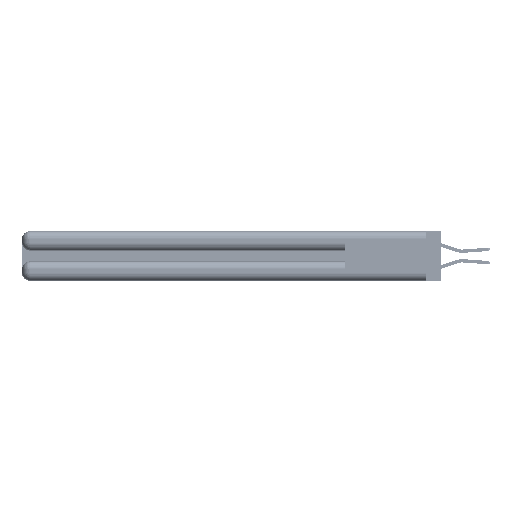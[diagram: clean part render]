
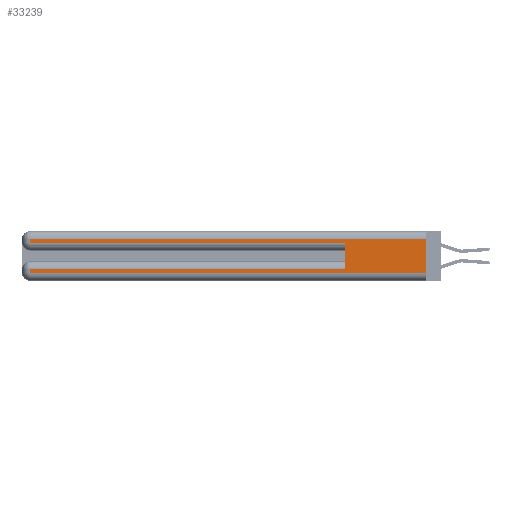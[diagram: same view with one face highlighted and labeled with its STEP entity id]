
A CAD part, left-side view. The second image highlights one B-rep face of the part: STEP entity #33239.
In plain terms, the highlighted planar face has unit normal (-1, 0, 0).
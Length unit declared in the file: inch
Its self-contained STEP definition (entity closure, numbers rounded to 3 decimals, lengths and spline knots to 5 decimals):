
#324 = LINE ( 'NONE', #23147, #6825 ) ;
#1380 = PLANE ( 'NONE',  #4083 ) ;
#4083 = AXIS2_PLACEMENT_3D ( 'NONE', #9706, #13821, #17948 ) ;
#4121 = CARTESIAN_POINT ( 'NONE',  ( 0., 0., 0.285 ) ) ;
#4352 = EDGE_CURVE ( 'NONE', #18697, #49655, #17958, .T. ) ;
#6003 = CARTESIAN_POINT ( 'NONE',  ( 0., 2.94, 0.085 ) ) ;
#6825 = VECTOR ( 'NONE', #51943, 39.37008 ) ;
#7717 = VERTEX_POINT ( 'NONE', #25868 ) ;
#7947 = LINE ( 'NONE', #16508, #23397 ) ;
#8087 = ORIENTED_EDGE ( 'NONE', *, *, #45344, .T. ) ;
#8477 = LINE ( 'NONE', #27884, #30405 ) ;
#9000 = VERTEX_POINT ( 'NONE', #42973 ) ;
#9706 = CARTESIAN_POINT ( 'NONE',  ( 0., 0., 0.37 ) ) ;
#9936 = VERTEX_POINT ( 'NONE', #25218 ) ;
#11226 = CARTESIAN_POINT ( 'NONE',  ( 0., 2.94, 0.285 ) ) ;
#11917 = DIRECTION ( 'NONE',  ( 0., 0., -1. ) ) ;
#12040 = ORIENTED_EDGE ( 'NONE', *, *, #44497, .T. ) ;
#12466 = EDGE_CURVE ( 'NONE', #9000, #18697, #31203, .T. ) ;
#12529 = EDGE_LOOP ( 'NONE', ( #28796, #12040, #33891, #22544, #28391, #52327, #8087, #31484 ) ) ;
#12564 = LINE ( 'NONE', #38827, #42848 ) ;
#13821 = DIRECTION ( 'NONE',  ( 1., 0., 0. ) ) ;
#16216 = CARTESIAN_POINT ( 'NONE',  ( 0., 2.94, 0.37 ) ) ;
#16252 = EDGE_CURVE ( 'NONE', #9936, #47673, #8477, .T. ) ;
#16508 = CARTESIAN_POINT ( 'NONE',  ( 0., 0.6, 0.145 ) ) ;
#17948 = DIRECTION ( 'NONE',  ( 0., 0., -1. ) ) ;
#17958 = LINE ( 'NONE', #4121, #23748 ) ;
#18697 = VERTEX_POINT ( 'NONE', #11226 ) ;
#19847 = LINE ( 'NONE', #52032, #21826 ) ;
#20217 = VECTOR ( 'NONE', #26576, 39.37008 ) ;
#21826 = VECTOR ( 'NONE', #31521, 39.37008 ) ;
#22544 = ORIENTED_EDGE ( 'NONE', *, *, #4352, .T. ) ;
#22994 = DIRECTION ( 'NONE',  ( 0., 1., 0. ) ) ;
#23147 = CARTESIAN_POINT ( 'NONE',  ( 0., 0., 0.085 ) ) ;
#23397 = VECTOR ( 'NONE', #37931, 39.37008 ) ;
#23748 = VECTOR ( 'NONE', #41397, 39.37008 ) ;
#25218 = CARTESIAN_POINT ( 'NONE',  ( 0., 0., 0.31 ) ) ;
#25563 = EDGE_CURVE ( 'NONE', #47698, #49655, #7947, .T. ) ;
#25868 = CARTESIAN_POINT ( 'NONE',  ( 0., 2.94, 0.06 ) ) ;
#26576 = DIRECTION ( 'NONE',  ( 0., 0., -1. ) ) ;
#27884 = CARTESIAN_POINT ( 'NONE',  ( 0., 0., 0.37 ) ) ;
#28391 = ORIENTED_EDGE ( 'NONE', *, *, #25563, .F. ) ;
#28796 = ORIENTED_EDGE ( 'NONE', *, *, #16252, .F. ) ;
#29294 = CARTESIAN_POINT ( 'NONE',  ( 0., 0.6, 0.085 ) ) ;
#30405 = VECTOR ( 'NONE', #48243, 39.37008 ) ;
#31203 = LINE ( 'NONE', #46912, #20217 ) ;
#31484 = ORIENTED_EDGE ( 'NONE', *, *, #49767, .T. ) ;
#31521 = DIRECTION ( 'NONE',  ( 0., -1., 0. ) ) ;
#32167 = EDGE_CURVE ( 'NONE', #47698, #36708, #324, .T. ) ;
#33239 = ADVANCED_FACE ( 'NONE', ( #45410 ), #1380, .F. ) ;
#33891 = ORIENTED_EDGE ( 'NONE', *, *, #12466, .T. ) ;
#36708 = VERTEX_POINT ( 'NONE', #6003 ) ;
#37908 = CARTESIAN_POINT ( 'NONE',  ( 0., 0., 0.06 ) ) ;
#37931 = DIRECTION ( 'NONE',  ( 0., 0., 1. ) ) ;
#38827 = CARTESIAN_POINT ( 'NONE',  ( 0., 0., 0.31 ) ) ;
#38896 = CARTESIAN_POINT ( 'NONE',  ( 0., 0.6, 0.285 ) ) ;
#41397 = DIRECTION ( 'NONE',  ( 0., -1., 0. ) ) ;
#42848 = VECTOR ( 'NONE', #22994, 39.37008 ) ;
#42973 = CARTESIAN_POINT ( 'NONE',  ( 0., 2.94, 0.31 ) ) ;
#44497 = EDGE_CURVE ( 'NONE', #9936, #9000, #12564, .T. ) ;
#45344 = EDGE_CURVE ( 'NONE', #36708, #7717, #51117, .T. ) ;
#45410 = FACE_OUTER_BOUND ( 'NONE', #12529, .T. ) ;
#46912 = CARTESIAN_POINT ( 'NONE',  ( 0., 2.94, 0.37 ) ) ;
#47673 = VERTEX_POINT ( 'NONE', #37908 ) ;
#47698 = VERTEX_POINT ( 'NONE', #29294 ) ;
#48243 = DIRECTION ( 'NONE',  ( 0., 0., -1. ) ) ;
#49655 = VERTEX_POINT ( 'NONE', #38896 ) ;
#49767 = EDGE_CURVE ( 'NONE', #7717, #47673, #19847, .T. ) ;
#51117 = LINE ( 'NONE', #16216, #53034 ) ;
#51943 = DIRECTION ( 'NONE',  ( 0., 1., 0. ) ) ;
#52032 = CARTESIAN_POINT ( 'NONE',  ( 0., 0., 0.06 ) ) ;
#52327 = ORIENTED_EDGE ( 'NONE', *, *, #32167, .T. ) ;
#53034 = VECTOR ( 'NONE', #11917, 39.37008 ) ;
